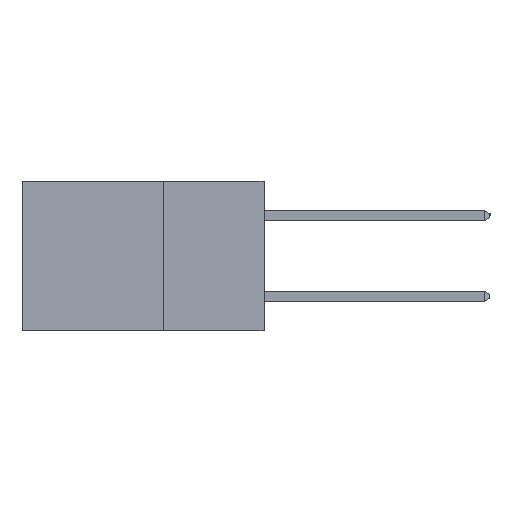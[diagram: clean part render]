
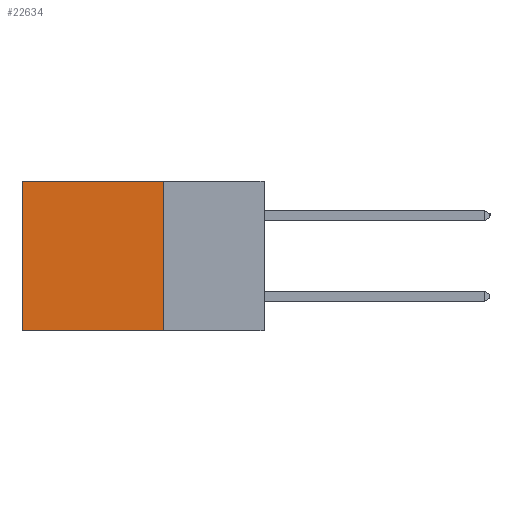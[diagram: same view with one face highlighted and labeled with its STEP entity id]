
A CAD part, left-side view. The second image highlights one B-rep face of the part: STEP entity #22634.
In plain terms, the highlighted planar face has unit normal (-1, 0, 0).
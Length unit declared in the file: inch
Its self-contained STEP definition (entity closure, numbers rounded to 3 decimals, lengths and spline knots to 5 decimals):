
#86 = DIRECTION ( 'NONE',  ( 1., 0., 0. ) ) ;
#274 = EDGE_CURVE ( 'NONE', #19860, #15870, #19798, .T. ) ;
#651 = ORIENTED_EDGE ( 'NONE', *, *, #10158, .F. ) ;
#726 = EDGE_CURVE ( 'NONE', #12014, #15870, #14352, .T. ) ;
#1597 = DIRECTION ( 'NONE',  ( 0., 1., 0. ) ) ;
#2312 = CARTESIAN_POINT ( 'NONE',  ( 0.2615, 0.25, -0.37 ) ) ;
#3132 = ORIENTED_EDGE ( 'NONE', *, *, #726, .F. ) ;
#3196 = VECTOR ( 'NONE', #10364, 39.37008 ) ;
#3635 = EDGE_CURVE ( 'NONE', #3725, #19860, #21148, .T. ) ;
#3725 = VERTEX_POINT ( 'NONE', #14398 ) ;
#4246 = ORIENTED_EDGE ( 'NONE', *, *, #3635, .T. ) ;
#5066 = VECTOR ( 'NONE', #1597, 39.37008 ) ;
#5080 = CARTESIAN_POINT ( 'NONE',  ( 0.2615, 0.6, -0.37 ) ) ;
#5572 = DIRECTION ( 'NONE',  ( 0., 0., -1. ) ) ;
#8155 = DIRECTION ( 'NONE',  ( 0., 0., -1. ) ) ;
#9152 = PLANE ( 'NONE',  #21798 ) ;
#9510 = CARTESIAN_POINT ( 'NONE',  ( 0.2615, 0.6, -0.37 ) ) ;
#10158 = EDGE_CURVE ( 'NONE', #3725, #12014, #16731, .T. ) ;
#10364 = DIRECTION ( 'NONE',  ( 0., 1., 0. ) ) ;
#10592 = DIRECTION ( 'NONE',  ( 0., 0., -1. ) ) ;
#12014 = VERTEX_POINT ( 'NONE', #21024 ) ;
#13933 = CARTESIAN_POINT ( 'NONE',  ( 0.2615, 0.25, 0. ) ) ;
#14352 = LINE ( 'NONE', #19420, #5066 ) ;
#14398 = CARTESIAN_POINT ( 'NONE',  ( 0.2615, 0.25, 0. ) ) ;
#15614 = ORIENTED_EDGE ( 'NONE', *, *, #274, .T. ) ;
#15870 = VERTEX_POINT ( 'NONE', #9510 ) ;
#16404 = CARTESIAN_POINT ( 'NONE',  ( 0.2615, 0.25, -0.37 ) ) ;
#16731 = LINE ( 'NONE', #2312, #21348 ) ;
#17474 = CARTESIAN_POINT ( 'NONE',  ( 0.2615, 0.6, 0. ) ) ;
#18087 = VECTOR ( 'NONE', #10592, 39.37008 ) ;
#19420 = CARTESIAN_POINT ( 'NONE',  ( 0.2615, 0.25, -0.37 ) ) ;
#19798 = LINE ( 'NONE', #5080, #18087 ) ;
#19860 = VERTEX_POINT ( 'NONE', #17474 ) ;
#19929 = FACE_OUTER_BOUND ( 'NONE', #22960, .T. ) ;
#21024 = CARTESIAN_POINT ( 'NONE',  ( 0.2615, 0.25, -0.37 ) ) ;
#21148 = LINE ( 'NONE', #13933, #3196 ) ;
#21348 = VECTOR ( 'NONE', #8155, 39.37008 ) ;
#21798 = AXIS2_PLACEMENT_3D ( 'NONE', #16404, #86, #5572 ) ;
#22634 = ADVANCED_FACE ( 'NONE', ( #19929 ), #9152, .F. ) ;
#22960 = EDGE_LOOP ( 'NONE', ( #15614, #3132, #651, #4246 ) ) ;
